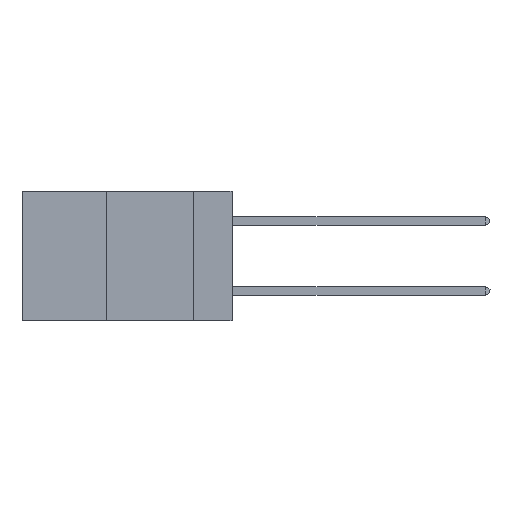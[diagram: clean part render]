
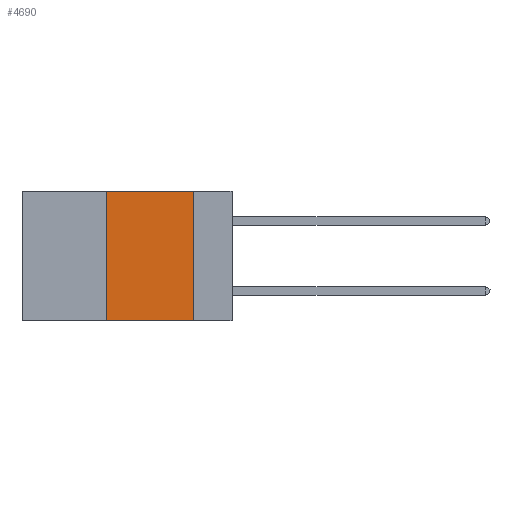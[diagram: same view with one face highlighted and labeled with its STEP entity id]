
A CAD part, left-side view. The second image highlights one B-rep face of the part: STEP entity #4690.
In plain terms, the highlighted planar face has unit normal (-1, 0, 0).
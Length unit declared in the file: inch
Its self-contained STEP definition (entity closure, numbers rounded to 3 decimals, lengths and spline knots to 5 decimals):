
#478 = ORIENTED_EDGE ( 'NONE', *, *, #2027, .F. ) ;
#502 = EDGE_CURVE ( 'NONE', #6314, #10281, #6291, .T. ) ;
#633 = DIRECTION ( 'NONE',  ( 0., 0., -1. ) ) ;
#2027 = EDGE_CURVE ( 'NONE', #10949, #6314, #13015, .T. ) ;
#2385 = CARTESIAN_POINT ( 'NONE',  ( 0., 0.6, -0.37 ) ) ;
#3573 = CARTESIAN_POINT ( 'NONE',  ( 0., 0.6, 0. ) ) ;
#3814 = CARTESIAN_POINT ( 'NONE',  ( 0., 0.36, -0.37 ) ) ;
#4690 = ADVANCED_FACE ( 'NONE', ( #17448 ), #11105, .F. ) ;
#5766 = CARTESIAN_POINT ( 'NONE',  ( 0., 0.36, 0. ) ) ;
#6060 = CARTESIAN_POINT ( 'NONE',  ( 0., 0.11, 0. ) ) ;
#6291 = LINE ( 'NONE', #7918, #10185 ) ;
#6303 = LINE ( 'NONE', #2385, #7892 ) ;
#6314 = VERTEX_POINT ( 'NONE', #6060 ) ;
#7541 = ORIENTED_EDGE ( 'NONE', *, *, #502, .F. ) ;
#7892 = VECTOR ( 'NONE', #9894, 39.37008 ) ;
#7918 = CARTESIAN_POINT ( 'NONE',  ( 0., 0.11, 0. ) ) ;
#8014 = EDGE_CURVE ( 'NONE', #13424, #10281, #6303, .T. ) ;
#8199 = DIRECTION ( 'NONE',  ( 1., 0., 0. ) ) ;
#8514 = VECTOR ( 'NONE', #16587, 39.37008 ) ;
#9548 = LINE ( 'NONE', #5766, #13168 ) ;
#9886 = AXIS2_PLACEMENT_3D ( 'NONE', #12723, #8199, #18347 ) ;
#9894 = DIRECTION ( 'NONE',  ( 0., -1., 0. ) ) ;
#10185 = VECTOR ( 'NONE', #633, 39.37008 ) ;
#10281 = VERTEX_POINT ( 'NONE', #11981 ) ;
#10949 = VERTEX_POINT ( 'NONE', #12362 ) ;
#11105 = PLANE ( 'NONE',  #9886 ) ;
#11981 = CARTESIAN_POINT ( 'NONE',  ( 0., 0.11, -0.37 ) ) ;
#12362 = CARTESIAN_POINT ( 'NONE',  ( 0., 0.36, 0. ) ) ;
#12723 = CARTESIAN_POINT ( 'NONE',  ( 0., 0.6, 0. ) ) ;
#13015 = LINE ( 'NONE', #3573, #8514 ) ;
#13168 = VECTOR ( 'NONE', #15843, 39.37008 ) ;
#13424 = VERTEX_POINT ( 'NONE', #3814 ) ;
#13853 = EDGE_LOOP ( 'NONE', ( #7541, #478, #14058, #16421 ) ) ;
#14058 = ORIENTED_EDGE ( 'NONE', *, *, #16858, .F. ) ;
#15843 = DIRECTION ( 'NONE',  ( 0., 0., 1. ) ) ;
#16421 = ORIENTED_EDGE ( 'NONE', *, *, #8014, .T. ) ;
#16587 = DIRECTION ( 'NONE',  ( 0., -1., 0. ) ) ;
#16858 = EDGE_CURVE ( 'NONE', #13424, #10949, #9548, .T. ) ;
#17448 = FACE_OUTER_BOUND ( 'NONE', #13853, .T. ) ;
#18347 = DIRECTION ( 'NONE',  ( 0., 0., -1. ) ) ;
